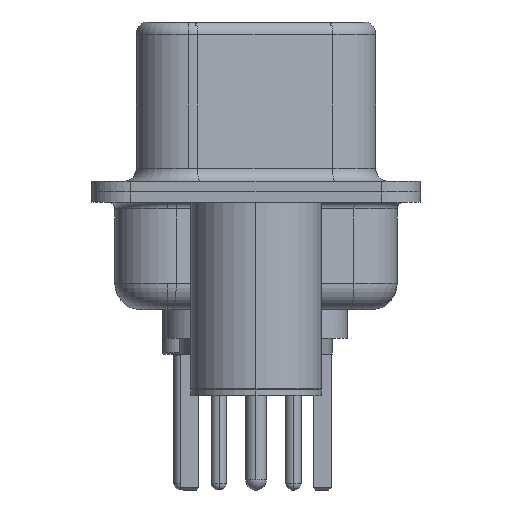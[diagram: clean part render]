
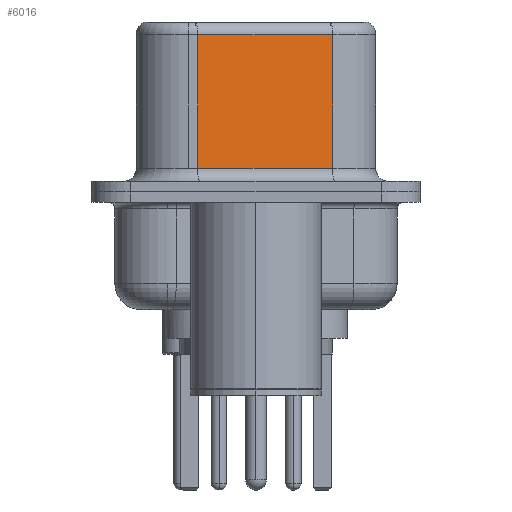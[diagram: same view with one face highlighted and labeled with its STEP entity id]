
A CAD part, left-side view. The second image highlights one B-rep face of the part: STEP entity #6016.
In plain terms, the highlighted planar face has unit normal (-0.985, -0.174, 0).
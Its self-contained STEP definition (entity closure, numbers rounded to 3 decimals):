
#146 = ORIENTED_EDGE ( 'NONE', *, *, #6030, .T. ) ;
#590 = DIRECTION ( 'NONE',  ( 0.174, -0.985, 0. ) ) ;
#1219 = VECTOR ( 'NONE', #12050, 1000. ) ;
#1555 = LINE ( 'NONE', #14952, #7046 ) ;
#1611 = VECTOR ( 'NONE', #590, 1000. ) ;
#4559 = DIRECTION ( 'NONE',  ( 0., 0., -1. ) ) ;
#4600 = CARTESIAN_POINT ( 'NONE',  ( 4.58, -2.927, 6.52 ) ) ;
#5313 = LINE ( 'NONE', #19213, #25584 ) ;
#5641 = CARTESIAN_POINT ( 'NONE',  ( 3.67, 2.233, 0.9 ) ) ;
#6016 = ADVANCED_FACE ( 'NONE', ( #7718 ), #10799, .F. ) ;
#6030 = EDGE_CURVE ( 'NONE', #20964, #9792, #7098, .T. ) ;
#6742 = LINE ( 'NONE', #16300, #1219 ) ;
#7046 = VECTOR ( 'NONE', #8760, 1000. ) ;
#7098 = LINE ( 'NONE', #8836, #1611 ) ;
#7718 = FACE_OUTER_BOUND ( 'NONE', #19727, .T. ) ;
#8541 = AXIS2_PLACEMENT_3D ( 'NONE', #4600, #25535, #12929 ) ;
#8760 = DIRECTION ( 'NONE',  ( -0.174, 0.985, 0. ) ) ;
#8836 = CARTESIAN_POINT ( 'NONE',  ( 4.58, -2.927, 0.9 ) ) ;
#9792 = VERTEX_POINT ( 'NONE', #15818 ) ;
#10799 = PLANE ( 'NONE',  #8541 ) ;
#11540 = EDGE_CURVE ( 'NONE', #25351, #9792, #5313, .T. ) ;
#11760 = CARTESIAN_POINT ( 'NONE',  ( 4.58, -2.927, 6.02 ) ) ;
#12050 = DIRECTION ( 'NONE',  ( 0., 0., -1. ) ) ;
#12929 = DIRECTION ( 'NONE',  ( -0.174, 0.985, 0. ) ) ;
#13088 = CARTESIAN_POINT ( 'NONE',  ( 3.67, 2.233, 6.02 ) ) ;
#14952 = CARTESIAN_POINT ( 'NONE',  ( 4.58, -2.927, 6.02 ) ) ;
#15818 = CARTESIAN_POINT ( 'NONE',  ( 4.58, -2.927, 0.9 ) ) ;
#16300 = CARTESIAN_POINT ( 'NONE',  ( 3.67, 2.233, 6.52 ) ) ;
#17297 = ORIENTED_EDGE ( 'NONE', *, *, #18124, .T. ) ;
#17819 = EDGE_CURVE ( 'NONE', #21390, #20964, #6742, .T. ) ;
#18124 = EDGE_CURVE ( 'NONE', #25351, #21390, #1555, .T. ) ;
#18887 = ORIENTED_EDGE ( 'NONE', *, *, #17819, .T. ) ;
#19213 = CARTESIAN_POINT ( 'NONE',  ( 4.58, -2.927, 6.52 ) ) ;
#19712 = ORIENTED_EDGE ( 'NONE', *, *, #11540, .F. ) ;
#19727 = EDGE_LOOP ( 'NONE', ( #19712, #17297, #18887, #146 ) ) ;
#20964 = VERTEX_POINT ( 'NONE', #5641 ) ;
#21390 = VERTEX_POINT ( 'NONE', #13088 ) ;
#25351 = VERTEX_POINT ( 'NONE', #11760 ) ;
#25535 = DIRECTION ( 'NONE',  ( 0.985, 0.174, 0. ) ) ;
#25584 = VECTOR ( 'NONE', #4559, 1000. ) ;
